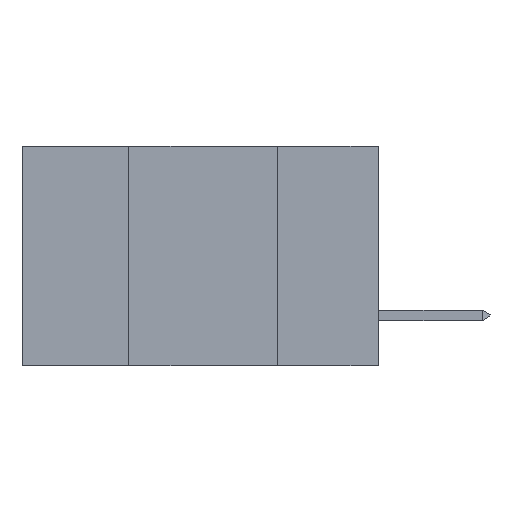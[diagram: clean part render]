
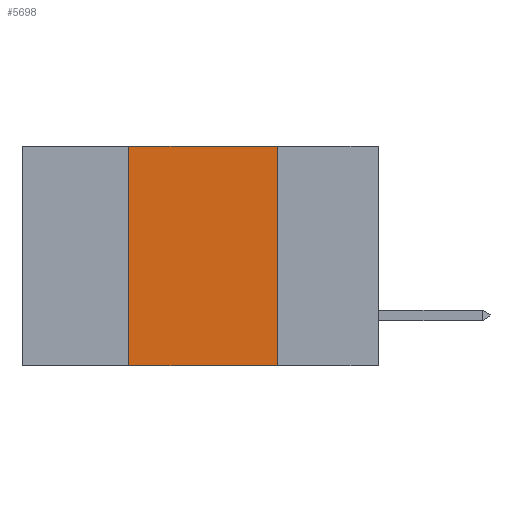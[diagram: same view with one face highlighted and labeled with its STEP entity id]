
A CAD part, left-side view. The second image highlights one B-rep face of the part: STEP entity #5698.
In plain terms, the highlighted planar face has unit normal (-1, 0, 0).
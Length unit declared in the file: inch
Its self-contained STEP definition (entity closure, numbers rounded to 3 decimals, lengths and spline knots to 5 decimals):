
#170 = DIRECTION ( 'NONE',  ( 0., 0., -1. ) ) ;
#631 = VERTEX_POINT ( 'NONE', #7283 ) ;
#665 = VERTEX_POINT ( 'NONE', #7222 ) ;
#899 = EDGE_CURVE ( 'NONE', #5795, #5664, #2178, .T. ) ;
#1812 = CARTESIAN_POINT ( 'NONE',  ( 0., 0.42, 0. ) ) ;
#2027 = LINE ( 'NONE', #5488, #2858 ) ;
#2178 = LINE ( 'NONE', #9248, #7325 ) ;
#2288 = VECTOR ( 'NONE', #3402, 39.37008 ) ;
#2482 = CARTESIAN_POINT ( 'NONE',  ( 0., 0.6, 0. ) ) ;
#2858 = VECTOR ( 'NONE', #3927, 39.37008 ) ;
#3159 = EDGE_LOOP ( 'NONE', ( #3297, #4369, #4405, #6285 ) ) ;
#3297 = ORIENTED_EDGE ( 'NONE', *, *, #899, .F. ) ;
#3402 = DIRECTION ( 'NONE',  ( 0., 0., 1. ) ) ;
#3521 = LINE ( 'NONE', #9448, #4480 ) ;
#3927 = DIRECTION ( 'NONE',  ( 0., -1., 0. ) ) ;
#4004 = DIRECTION ( 'NONE',  ( 0., -1., 0. ) ) ;
#4043 = DIRECTION ( 'NONE',  ( 1., 0., 0. ) ) ;
#4369 = ORIENTED_EDGE ( 'NONE', *, *, #7377, .F. ) ;
#4405 = ORIENTED_EDGE ( 'NONE', *, *, #5789, .F. ) ;
#4480 = VECTOR ( 'NONE', #4004, 39.37008 ) ;
#4719 = CARTESIAN_POINT ( 'NONE',  ( 0., 0.17, -0.37 ) ) ;
#4901 = EDGE_CURVE ( 'NONE', #631, #5664, #3521, .T. ) ;
#5488 = CARTESIAN_POINT ( 'NONE',  ( 0., 0.6, 0. ) ) ;
#5548 = LINE ( 'NONE', #1812, #2288 ) ;
#5664 = VERTEX_POINT ( 'NONE', #4719 ) ;
#5698 = ADVANCED_FACE ( 'NONE', ( #8409 ), #7084, .F. ) ;
#5789 = EDGE_CURVE ( 'NONE', #631, #665, #5548, .T. ) ;
#5795 = VERTEX_POINT ( 'NONE', #9526 ) ;
#6285 = ORIENTED_EDGE ( 'NONE', *, *, #4901, .T. ) ;
#7084 = PLANE ( 'NONE',  #7211 ) ;
#7211 = AXIS2_PLACEMENT_3D ( 'NONE', #2482, #4043, #170 ) ;
#7222 = CARTESIAN_POINT ( 'NONE',  ( 0., 0.42, 0. ) ) ;
#7283 = CARTESIAN_POINT ( 'NONE',  ( 0., 0.42, -0.37 ) ) ;
#7325 = VECTOR ( 'NONE', #8361, 39.37008 ) ;
#7377 = EDGE_CURVE ( 'NONE', #665, #5795, #2027, .T. ) ;
#8361 = DIRECTION ( 'NONE',  ( 0., 0., -1. ) ) ;
#8409 = FACE_OUTER_BOUND ( 'NONE', #3159, .T. ) ;
#9248 = CARTESIAN_POINT ( 'NONE',  ( 0., 0.17, 0. ) ) ;
#9448 = CARTESIAN_POINT ( 'NONE',  ( 0., 0.6, -0.37 ) ) ;
#9526 = CARTESIAN_POINT ( 'NONE',  ( 0., 0.17, 0. ) ) ;
